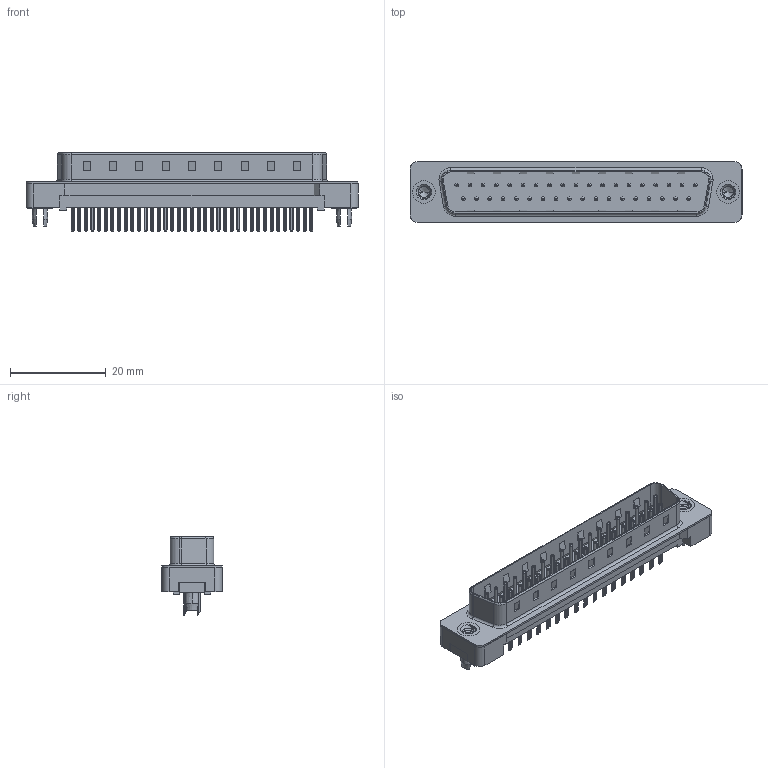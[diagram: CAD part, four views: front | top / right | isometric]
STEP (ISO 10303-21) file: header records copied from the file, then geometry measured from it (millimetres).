
FILE_DESCRIPTION (( 'STEP AP203' ), '1' );
FILE_NAME ('627-037-224-216.STEP', '2020-07-16T01:42:26', ( '' ), ( '' ), 'SwSTEP 2.0', 'SolidWorks 2020', '' );
FILE_SCHEMA (( 'CONFIG_CONTROL_DESIGN' ));
Length unit declared in the file: millimetre
Products named in the file (6): 627-037-224-216; 627 PB Contact Row 2_24; 627 PB Contact Row 1_24; 627 PB 4-40 Threaded Rivet with Boardlock; 627 Plastic Body Housing_37 Contacts; 627 PB Shell_37 Contacts
Assembly tree (41 placements, depth 2):
  627-037-224-216
    627 Plastic Body Housing_37 Contacts
    627 PB Shell_37 Contacts
    627 PB Contact Row 1_24  x19
    627 PB Contact Row 2_24  x18
    627 PB 4-40 Threaded Rivet with Boardlock  x2
Bounding box: 69.32 x 12.6 x 16.3 mm (x, y, z)
Volume: 3250.6 mm3; surface area: 7837.3 mm2
Topology: 41 solids, 41 shells, 2503 faces, 6652 edges, 4281 vertices
Faces by surface type: plane 1651, cylinder 694, torus 130, cone 22, bspline 6
Entity records: 29146 total; most frequent: CARTESIAN_POINT 5655, DIRECTION 4541, ORIENTED_EDGE 4528, EDGE_CURVE 2264, LINE 1657, VECTOR 1657, VERTEX_POINT 1476, AXIS2_PLACEMENT_3D 1442
